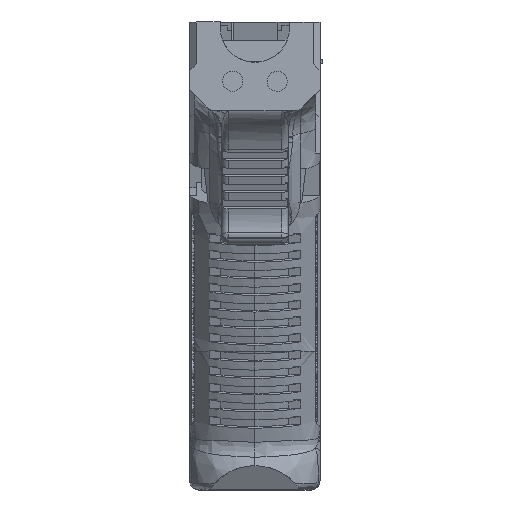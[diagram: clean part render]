
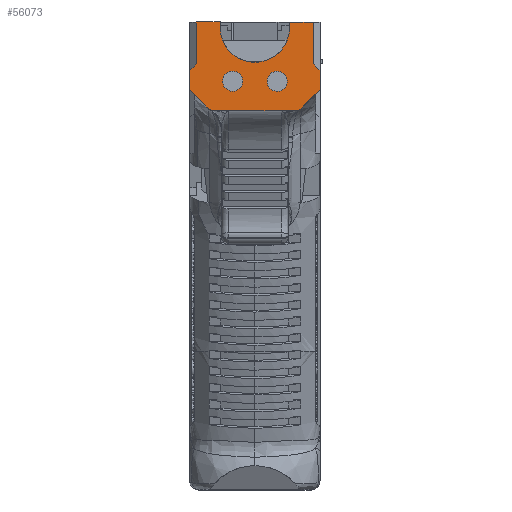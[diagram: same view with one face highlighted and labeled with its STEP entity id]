
A CAD part, left-side view. The second image highlights one B-rep face of the part: STEP entity #56073.
In plain terms, the highlighted planar face has unit normal (-1, 0, 0).
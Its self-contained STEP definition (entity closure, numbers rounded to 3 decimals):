
#7398=FACE_BOUND('',#11213,.T.);
#7399=FACE_BOUND('',#11214,.T.);
#7821=FACE_OUTER_BOUND('',#11212,.T.);
#11212=EDGE_LOOP('',(#37276,#37277,#37278,#37279,#37280,#37281,#37282,#37283,
#37284,#37285,#37286,#37287,#37288,#37289,#37290,#37291));
#11213=EDGE_LOOP('',(#37292));
#11214=EDGE_LOOP('',(#37293));
#15026=LINE('',#67191,#18658);
#15027=LINE('',#67193,#18659);
#15028=LINE('',#67195,#18660);
#15029=LINE('',#67197,#18661);
#15030=LINE('',#67199,#18662);
#15031=LINE('',#67201,#18663);
#15032=LINE('',#67205,#18664);
#15033=LINE('',#67209,#18665);
#15034=LINE('',#67211,#18666);
#15035=LINE('',#67213,#18667);
#15036=LINE('',#67215,#18668);
#15037=LINE('',#67217,#18669);
#15038=LINE('',#67218,#18670);
#18658=VECTOR('',#60835,10.);
#18659=VECTOR('',#60836,10.);
#18660=VECTOR('',#60837,10.);
#18661=VECTOR('',#60838,10.);
#18662=VECTOR('',#60839,10.);
#18663=VECTOR('',#60840,10.);
#18664=VECTOR('',#60843,10.);
#18665=VECTOR('',#60846,10.);
#18666=VECTOR('',#60847,10.);
#18667=VECTOR('',#60848,10.);
#18668=VECTOR('',#60849,10.);
#18669=VECTOR('',#60850,10.);
#18670=VECTOR('',#60851,10.);
#22290=CIRCLE('',#59469,7.765);
#22291=CIRCLE('',#59470,3.);
#22292=CIRCLE('',#59471,3.);
#22293=CIRCLE('',#59472,2.25);
#22294=CIRCLE('',#59473,2.25);
#22512=VERTEX_POINT('',#67187);
#22513=VERTEX_POINT('',#67188);
#22514=VERTEX_POINT('',#67190);
#22515=VERTEX_POINT('',#67192);
#22516=VERTEX_POINT('',#67194);
#22517=VERTEX_POINT('',#67196);
#22518=VERTEX_POINT('',#67198);
#22519=VERTEX_POINT('',#67200);
#22520=VERTEX_POINT('',#67202);
#22521=VERTEX_POINT('',#67204);
#22522=VERTEX_POINT('',#67206);
#22523=VERTEX_POINT('',#67208);
#22524=VERTEX_POINT('',#67210);
#22525=VERTEX_POINT('',#67212);
#22526=VERTEX_POINT('',#67214);
#22527=VERTEX_POINT('',#67216);
#22528=VERTEX_POINT('',#67219);
#22529=VERTEX_POINT('',#67221);
#28395=EDGE_CURVE('',#22512,#22513,#22290,.T.);
#28396=EDGE_CURVE('',#22512,#22514,#15026,.T.);
#28397=EDGE_CURVE('',#22514,#22515,#15027,.T.);
#28398=EDGE_CURVE('',#22515,#22516,#15028,.T.);
#28399=EDGE_CURVE('',#22516,#22517,#15029,.T.);
#28400=EDGE_CURVE('',#22517,#22518,#15030,.T.);
#28401=EDGE_CURVE('',#22518,#22519,#15031,.T.);
#28402=EDGE_CURVE('',#22519,#22520,#22291,.T.);
#28403=EDGE_CURVE('',#22520,#22521,#15032,.T.);
#28404=EDGE_CURVE('',#22521,#22522,#22292,.T.);
#28405=EDGE_CURVE('',#22522,#22523,#15033,.T.);
#28406=EDGE_CURVE('',#22523,#22524,#15034,.T.);
#28407=EDGE_CURVE('',#22524,#22525,#15035,.T.);
#28408=EDGE_CURVE('',#22525,#22526,#15036,.T.);
#28409=EDGE_CURVE('',#22526,#22527,#15037,.T.);
#28410=EDGE_CURVE('',#22527,#22513,#15038,.T.);
#28411=EDGE_CURVE('',#22528,#22528,#22293,.T.);
#28412=EDGE_CURVE('',#22529,#22529,#22294,.T.);
#37276=ORIENTED_EDGE('',*,*,#28395,.F.);
#37277=ORIENTED_EDGE('',*,*,#28396,.T.);
#37278=ORIENTED_EDGE('',*,*,#28397,.T.);
#37279=ORIENTED_EDGE('',*,*,#28398,.T.);
#37280=ORIENTED_EDGE('',*,*,#28399,.T.);
#37281=ORIENTED_EDGE('',*,*,#28400,.T.);
#37282=ORIENTED_EDGE('',*,*,#28401,.T.);
#37283=ORIENTED_EDGE('',*,*,#28402,.T.);
#37284=ORIENTED_EDGE('',*,*,#28403,.T.);
#37285=ORIENTED_EDGE('',*,*,#28404,.T.);
#37286=ORIENTED_EDGE('',*,*,#28405,.T.);
#37287=ORIENTED_EDGE('',*,*,#28406,.T.);
#37288=ORIENTED_EDGE('',*,*,#28407,.T.);
#37289=ORIENTED_EDGE('',*,*,#28408,.T.);
#37290=ORIENTED_EDGE('',*,*,#28409,.T.);
#37291=ORIENTED_EDGE('',*,*,#28410,.T.);
#37292=ORIENTED_EDGE('',*,*,#28411,.T.);
#37293=ORIENTED_EDGE('',*,*,#28412,.T.);
#55038=PLANE('',#59468);
#56073=ADVANCED_FACE('',(#7821,#7398,#7399),#55038,.F.);
#59468=AXIS2_PLACEMENT_3D('',#67186,#60831,#60832);
#59469=AXIS2_PLACEMENT_3D('',#67189,#60833,#60834);
#59470=AXIS2_PLACEMENT_3D('',#67203,#60841,#60842);
#59471=AXIS2_PLACEMENT_3D('',#67207,#60844,#60845);
#59472=AXIS2_PLACEMENT_3D('',#67220,#60852,#60853);
#59473=AXIS2_PLACEMENT_3D('',#67222,#60854,#60855);
#60831=DIRECTION('center_axis',(1.,0.,0.));
#60832=DIRECTION('ref_axis',(0.,1.,0.));
#60833=DIRECTION('center_axis',(-1.,0.,0.));
#60834=DIRECTION('ref_axis',(0.,0.,
-1.));
#60835=DIRECTION('',(0.,0.,1.));
#60836=DIRECTION('',(0.,1.,0.));
#60837=DIRECTION('',(0.,0.,-1.));
#60838=DIRECTION('',(0.,0.707,-0.707));
#60839=DIRECTION('',(0.,0.,-1.));
#60840=DIRECTION('',(0.,-0.707,-0.707));
#60841=DIRECTION('center_axis',(-1.,0.,0.));
#60842=DIRECTION('ref_axis',(0.,0.383,-0.924));
#60843=DIRECTION('',(0.,-1.,0.));
#60844=DIRECTION('center_axis',(-1.,0.,0.));
#60845=DIRECTION('ref_axis',(0.,-0.383,-0.924));
#60846=DIRECTION('',(0.,-0.707,0.707));
#60847=DIRECTION('',(0.,0.,1.));
#60848=DIRECTION('',(0.,0.707,0.707));
#60849=DIRECTION('',(0.,0.,1.));
#60850=DIRECTION('',(0.,1.,0.));
#60851=DIRECTION('',(0.,0.,-1.));
#60852=DIRECTION('center_axis',(1.,0.,0.));
#60853=DIRECTION('ref_axis',(0.,0.726,-0.688));
#60854=DIRECTION('center_axis',(1.,0.,0.));
#60855=DIRECTION('ref_axis',(0.,1.,0.));
#67186=CARTESIAN_POINT('Origin',(258.489,26.849,-316.648));
#67187=CARTESIAN_POINT('',(258.489,34.614,-265.477));
#67188=CARTESIAN_POINT('',(258.489,19.086,-265.477));
#67189=CARTESIAN_POINT('Origin',(258.489,26.85,-265.35));
#67190=CARTESIAN_POINT('',(258.489,34.614,-264.061));
#67191=CARTESIAN_POINT('',(258.489,34.614,-290.936));
#67192=CARTESIAN_POINT('',(258.489,39.966,-264.061));
#67193=CARTESIAN_POINT('',(258.489,19.237,-264.061));
#67194=CARTESIAN_POINT('',(258.489,39.966,-273.447));
#67195=CARTESIAN_POINT('',(258.489,39.966,-290.048));
#67196=CARTESIAN_POINT('',(258.489,41.466,-274.947));
#67197=CARTESIAN_POINT('',(258.489,47.862,-281.343));
#67198=CARTESIAN_POINT('',(258.489,41.466,-279.25));
#67199=CARTESIAN_POINT('',(258.489,41.466,-290.301));
#67200=CARTESIAN_POINT('',(258.489,37.595,-283.122));
#67201=CARTESIAN_POINT('',(258.489,27.275,-293.442));
#67202=CARTESIAN_POINT('',(258.489,35.473,-284.));
#67203=CARTESIAN_POINT('Origin',(258.489,35.473,-281.));
#67204=CARTESIAN_POINT('',(258.489,18.227,-284.));
#67205=CARTESIAN_POINT('',(258.489,26.85,-284.));
#67206=CARTESIAN_POINT('',(258.489,16.105,-283.122));
#67207=CARTESIAN_POINT('Origin',(258.489,18.227,-281.));
#67208=CARTESIAN_POINT('',(258.489,12.234,-279.25));
#67209=CARTESIAN_POINT('',(258.489,26.425,-293.441));
#67210=CARTESIAN_POINT('',(258.489,12.234,-274.947));
#67211=CARTESIAN_POINT('',(258.489,12.234,-290.301));
#67212=CARTESIAN_POINT('',(258.489,13.734,-273.447));
#67213=CARTESIAN_POINT('',(258.489,5.837,-281.343));
#67214=CARTESIAN_POINT('',(258.489,13.734,-264.061));
#67215=CARTESIAN_POINT('',(258.489,13.734,-295.048));
#67216=CARTESIAN_POINT('',(258.489,19.086,-264.061));
#67217=CARTESIAN_POINT('',(258.489,19.237,-264.061));
#67218=CARTESIAN_POINT('',(258.489,19.086,-290.936));
#67219=CARTESIAN_POINT('',(258.489,20.217,-275.798));
#67220=CARTESIAN_POINT('Origin',(258.489,21.85,-277.346));
#67221=CARTESIAN_POINT('',(258.489,29.6,-277.346));
#67222=CARTESIAN_POINT('Origin',(258.489,31.85,-277.346));
